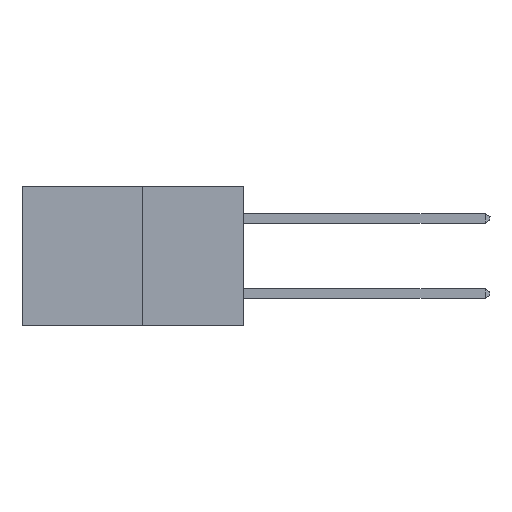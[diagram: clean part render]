
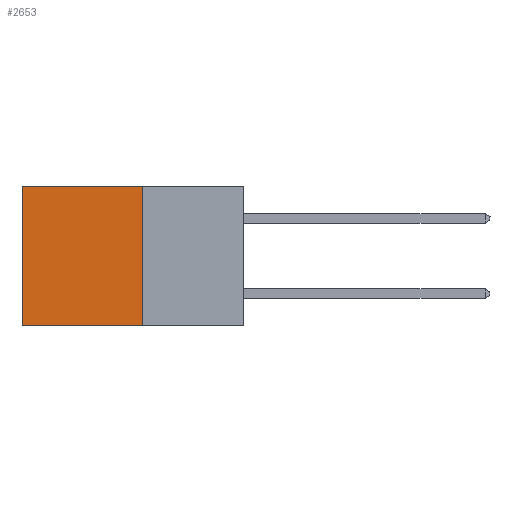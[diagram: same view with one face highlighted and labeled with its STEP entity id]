
A CAD part, left-side view. The second image highlights one B-rep face of the part: STEP entity #2653.
In plain terms, the highlighted planar face has unit normal (-1, 0, 0).
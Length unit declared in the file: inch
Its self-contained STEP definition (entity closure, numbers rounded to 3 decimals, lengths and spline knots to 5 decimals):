
#197 = CARTESIAN_POINT ( 'NONE',  ( 0.277, 0.27, 0. ) ) ;
#365 = CARTESIAN_POINT ( 'NONE',  ( 0.277, 0.27, -0.37 ) ) ;
#889 = VERTEX_POINT ( 'NONE', #197 ) ;
#1154 = EDGE_LOOP ( 'NONE', ( #17755, #6874, #14061, #16547 ) ) ;
#2203 = PLANE ( 'NONE',  #8509 ) ;
#2263 = VECTOR ( 'NONE', #3347, 39.37008 ) ;
#2297 = CARTESIAN_POINT ( 'NONE',  ( 0.277, 0.59, 0. ) ) ;
#2653 = ADVANCED_FACE ( 'NONE', ( #5133 ), #2203, .F. ) ;
#3004 = VERTEX_POINT ( 'NONE', #2297 ) ;
#3347 = DIRECTION ( 'NONE',  ( 0., 0., -1. ) ) ;
#4623 = CARTESIAN_POINT ( 'NONE',  ( 0.277, 0.59, -0.37 ) ) ;
#4780 = LINE ( 'NONE', #4942, #15542 ) ;
#4942 = CARTESIAN_POINT ( 'NONE',  ( 0.277, 0.59, -0.37 ) ) ;
#5133 = FACE_OUTER_BOUND ( 'NONE', #1154, .T. ) ;
#6261 = DIRECTION ( 'NONE',  ( 0., 0., -1. ) ) ;
#6482 = LINE ( 'NONE', #16365, #14280 ) ;
#6874 = ORIENTED_EDGE ( 'NONE', *, *, #11652, .F. ) ;
#7312 = EDGE_CURVE ( 'NONE', #3004, #17182, #4780, .T. ) ;
#8015 = DIRECTION ( 'NONE',  ( 1., 0., 0. ) ) ;
#8509 = AXIS2_PLACEMENT_3D ( 'NONE', #16720, #8015, #6261 ) ;
#8893 = EDGE_CURVE ( 'NONE', #889, #14763, #10055, .T. ) ;
#9535 = CARTESIAN_POINT ( 'NONE',  ( 0.277, 0.27, -0.37 ) ) ;
#10055 = LINE ( 'NONE', #365, #2263 ) ;
#10109 = CARTESIAN_POINT ( 'NONE',  ( 0.277, 0.27, 0. ) ) ;
#11652 = EDGE_CURVE ( 'NONE', #14763, #17182, #6482, .T. ) ;
#12719 = VECTOR ( 'NONE', #17411, 39.37008 ) ;
#13262 = EDGE_CURVE ( 'NONE', #889, #3004, #16553, .T. ) ;
#13530 = DIRECTION ( 'NONE',  ( 0., 1., 0. ) ) ;
#14061 = ORIENTED_EDGE ( 'NONE', *, *, #8893, .F. ) ;
#14280 = VECTOR ( 'NONE', #13530, 39.37008 ) ;
#14763 = VERTEX_POINT ( 'NONE', #9535 ) ;
#15542 = VECTOR ( 'NONE', #16950, 39.37008 ) ;
#16365 = CARTESIAN_POINT ( 'NONE',  ( 0.277, 0.27, -0.37 ) ) ;
#16547 = ORIENTED_EDGE ( 'NONE', *, *, #13262, .T. ) ;
#16553 = LINE ( 'NONE', #10109, #12719 ) ;
#16720 = CARTESIAN_POINT ( 'NONE',  ( 0.277, 0.27, -0.37 ) ) ;
#16950 = DIRECTION ( 'NONE',  ( 0., 0., -1. ) ) ;
#17182 = VERTEX_POINT ( 'NONE', #4623 ) ;
#17411 = DIRECTION ( 'NONE',  ( 0., 1., 0. ) ) ;
#17755 = ORIENTED_EDGE ( 'NONE', *, *, #7312, .T. ) ;
